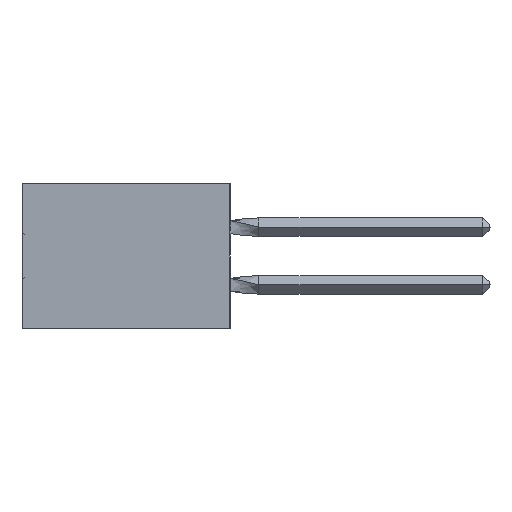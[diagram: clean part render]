
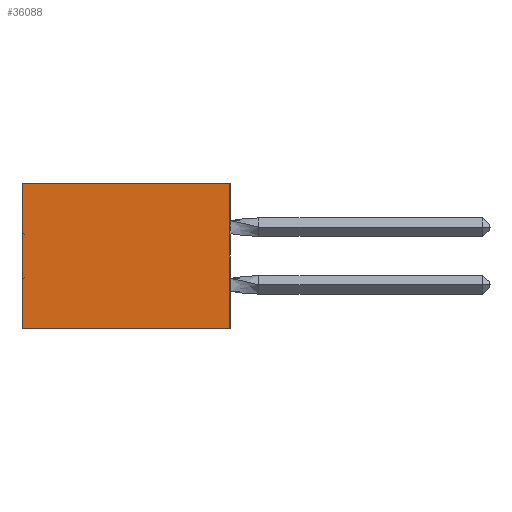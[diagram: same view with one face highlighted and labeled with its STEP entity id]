
A CAD part, left-side view. The second image highlights one B-rep face of the part: STEP entity #36088.
In plain terms, the highlighted planar face has unit normal (-1, 0, 0).
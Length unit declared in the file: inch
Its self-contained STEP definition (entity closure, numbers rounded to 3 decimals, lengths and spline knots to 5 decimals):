
#6357 = CARTESIAN_POINT ( 'NONE',  ( 0.305, 0., -0.5 ) ) ;
#7659 = LINE ( 'NONE', #14413, #54006 ) ;
#7884 = CARTESIAN_POINT ( 'NONE',  ( 0.305, 0., 0. ) ) ;
#9050 = EDGE_CURVE ( 'NONE', #30925, #17486, #29393, .T. ) ;
#9907 = ORIENTED_EDGE ( 'NONE', *, *, #41324, .F. ) ;
#10291 = VECTOR ( 'NONE', #53200, 39.37008 ) ;
#10397 = AXIS2_PLACEMENT_3D ( 'NONE', #6357, #33003, #55192 ) ;
#14413 = CARTESIAN_POINT ( 'NONE',  ( 0.305, 0.72, -0.5 ) ) ;
#15825 = EDGE_CURVE ( 'NONE', #30925, #34645, #31319, .T. ) ;
#17486 = VERTEX_POINT ( 'NONE', #54257 ) ;
#18595 = ORIENTED_EDGE ( 'NONE', *, *, #15825, .F. ) ;
#20683 = CARTESIAN_POINT ( 'NONE',  ( 0.305, 0., -0.5 ) ) ;
#24036 = CARTESIAN_POINT ( 'NONE',  ( 0.305, 0., -0.5 ) ) ;
#24039 = ORIENTED_EDGE ( 'NONE', *, *, #56350, .T. ) ;
#27437 = ORIENTED_EDGE ( 'NONE', *, *, #9050, .T. ) ;
#29393 = LINE ( 'NONE', #31367, #10291 ) ;
#29969 = VECTOR ( 'NONE', #41794, 39.37008 ) ;
#30925 = VERTEX_POINT ( 'NONE', #7884 ) ;
#31319 = LINE ( 'NONE', #20683, #29969 ) ;
#31367 = CARTESIAN_POINT ( 'NONE',  ( 0.305, 0., 0. ) ) ;
#31562 = VERTEX_POINT ( 'NONE', #46002 ) ;
#33003 = DIRECTION ( 'NONE',  ( 1., 0., 0. ) ) ;
#34645 = VERTEX_POINT ( 'NONE', #24036 ) ;
#34961 = LINE ( 'NONE', #48504, #47911 ) ;
#36088 = ADVANCED_FACE ( 'NONE', ( #43335 ), #54103, .F. ) ;
#41324 = EDGE_CURVE ( 'NONE', #34645, #31562, #34961, .T. ) ;
#41794 = DIRECTION ( 'NONE',  ( 0., 0., -1. ) ) ;
#43335 = FACE_OUTER_BOUND ( 'NONE', #55324, .T. ) ;
#46002 = CARTESIAN_POINT ( 'NONE',  ( 0.305, 0.72, -0.5 ) ) ;
#47911 = VECTOR ( 'NONE', #47947, 39.37008 ) ;
#47947 = DIRECTION ( 'NONE',  ( 0., 1., 0. ) ) ;
#48504 = CARTESIAN_POINT ( 'NONE',  ( 0.305, 0., -0.5 ) ) ;
#53027 = DIRECTION ( 'NONE',  ( 0., 0., -1. ) ) ;
#53200 = DIRECTION ( 'NONE',  ( 0., 1., 0. ) ) ;
#54006 = VECTOR ( 'NONE', #53027, 39.37008 ) ;
#54103 = PLANE ( 'NONE',  #10397 ) ;
#54257 = CARTESIAN_POINT ( 'NONE',  ( 0.305, 0.72, 0. ) ) ;
#55192 = DIRECTION ( 'NONE',  ( 0., 0., -1. ) ) ;
#55324 = EDGE_LOOP ( 'NONE', ( #24039, #9907, #18595, #27437 ) ) ;
#56350 = EDGE_CURVE ( 'NONE', #17486, #31562, #7659, .T. ) ;
